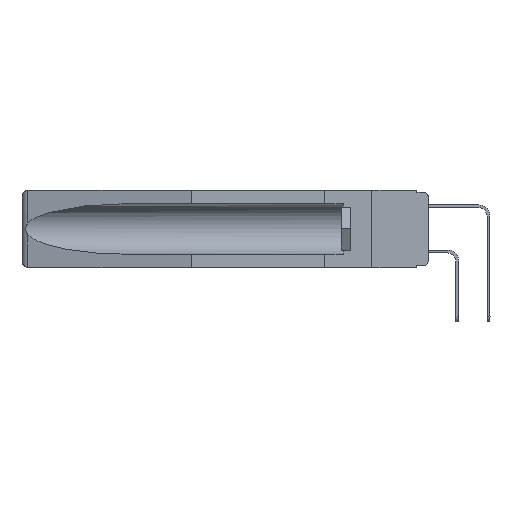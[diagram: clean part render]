
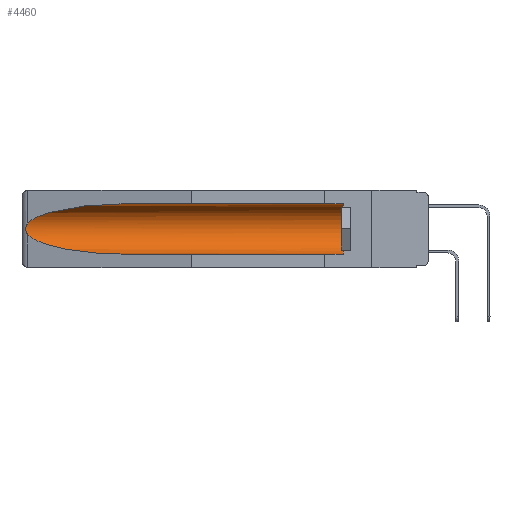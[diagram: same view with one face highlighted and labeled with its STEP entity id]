
A CAD part, left-side view. The second image highlights one B-rep face of the part: STEP entity #4460.
In plain terms, the highlighted cylindrical face has radius 2.857 mm (diameter 5.715 mm), a partial arc.
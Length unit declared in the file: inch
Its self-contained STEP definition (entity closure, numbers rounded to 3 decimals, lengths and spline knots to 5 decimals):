
#137 = DIRECTION ( 'NONE',  ( 0., -1., 0. ) ) ;
#471 = CARTESIAN_POINT ( 'NONE',  ( 0.2675, 1.53308, -0.17534 ) ) ;
#1247 = CARTESIAN_POINT ( 'NONE',  ( 0.25451, 1.48313, -0.24835 ) ) ;
#1530 = LINE ( 'NONE', #14724, #13781 ) ;
#1669 = CARTESIAN_POINT ( 'NONE',  ( 0.155, 0.126, -0.284 ) ) ;
#1723 = CARTESIAN_POINT ( 'NONE',  ( 0.2673, 1.53269, -0.17917 ) ) ;
#2307 = ORIENTED_EDGE ( 'NONE', *, *, #15177, .T. ) ;
#2541 = VERTEX_POINT ( 'NONE', #2817 ) ;
#2593 = VERTEX_POINT ( 'NONE', #18043 ) ;
#2817 = CARTESIAN_POINT ( 'NONE',  ( 0.26537, 1.52718, -0.14972 ) ) ;
#3163 = ORIENTED_EDGE ( 'NONE', *, *, #12112, .T. ) ;
#3260 = CARTESIAN_POINT ( 'NONE',  ( 0.155, 1.07973, -0.284 ) ) ;
#3589 = CYLINDRICAL_SURFACE ( 'NONE', #11812, 0.1125 ) ;
#3646 = CARTESIAN_POINT ( 'NONE',  ( 0.26597, 1.52961, -0.15275 ) ) ;
#3725 = ORIENTED_EDGE ( 'NONE', *, *, #11303, .T. ) ;
#4099 = CARTESIAN_POINT ( 'NONE',  ( 0.155, 1.07973, -0.059 ) ) ;
#4169 = EDGE_CURVE ( 'NONE', #15071, #11388, #14285, .T. ) ;
#4353 = AXIS2_PLACEMENT_3D ( 'NONE', #7747, #137, #16620 ) ;
#4460 = ADVANCED_FACE ( 'NONE', ( #13708 ), #3589, .F. ) ;
#4886 = CARTESIAN_POINT ( 'NONE',  ( 0.26537, 1.52718, -0.14972 ) ) ;
#4989 = CARTESIAN_POINT ( 'NONE',  ( 0.2675, 1.53308, -0.16763 ) ) ;
#5112 = EDGE_CURVE ( 'NONE', #15531, #12094, #1530, .T. ) ;
#5751 = DIRECTION ( 'NONE',  ( 0., 1., 0. ) ) ;
#5797 = CARTESIAN_POINT ( 'NONE',  ( 0.155, -0.30754, -0.284 ) ) ;
#6389 = CARTESIAN_POINT ( 'NONE',  ( 0.155, 1.07973, -0.059 ) ) ;
#6441 = CARTESIAN_POINT ( 'NONE',  ( 0.26654, 1.53092, -0.15636 ) ) ;
#6485 =( BOUNDED_CURVE ( )  B_SPLINE_CURVE ( 3, ( #4099, #12782, #17315, #12501 ),
 .UNSPECIFIED., .F., .F. ) 
 B_SPLINE_CURVE_WITH_KNOTS ( ( 4, 4 ),
 ( 4.71239, 6.08839 ),
 .UNSPECIFIED. ) 
 CURVE ( )  GEOMETRIC_REPRESENTATION_ITEM ( )  RATIONAL_B_SPLINE_CURVE ( ( 1., 0.848, 0.848, 1. ) ) 
 REPRESENTATION_ITEM ( '' )  );
#6518 = CIRCLE ( 'NONE', #4353, 0.1125 ) ;
#6541 = CARTESIAN_POINT ( 'NONE',  ( 0.2673, 1.5327, -0.16383 ) ) ;
#6859 = EDGE_LOOP ( 'NONE', ( #13386, #3725, #2307, #12552, #3163, #13947 ) ) ;
#7354 = DIRECTION ( 'NONE',  ( 0., 1., 0. ) ) ;
#7615 = VECTOR ( 'NONE', #7354, 39.37008 ) ;
#7747 = CARTESIAN_POINT ( 'NONE',  ( 0.155, 0.126, -0.1715 ) ) ;
#7890 = CARTESIAN_POINT ( 'NONE',  ( 0.26597, 1.5296, -0.19026 ) ) ;
#8590 = CARTESIAN_POINT ( 'NONE',  ( 0.155, 0.126, -0.059 ) ) ;
#11303 = EDGE_CURVE ( 'NONE', #2541, #2593, #15389, .T. ) ;
#11388 = VERTEX_POINT ( 'NONE', #3260 ) ;
#11812 = AXIS2_PLACEMENT_3D ( 'NONE', #15251, #15345, #16895 ) ;
#12094 = VERTEX_POINT ( 'NONE', #6389 ) ;
#12112 = EDGE_CURVE ( 'NONE', #15071, #15531, #6518, .T. ) ;
#12426 = CARTESIAN_POINT ( 'NONE',  ( 0.26655, 1.53094, -0.18657 ) ) ;
#12501 = CARTESIAN_POINT ( 'NONE',  ( 0.26537, 1.52718, -0.14972 ) ) ;
#12552 = ORIENTED_EDGE ( 'NONE', *, *, #4169, .F. ) ;
#12782 = CARTESIAN_POINT ( 'NONE',  ( 0.21114, 1.30732, -0.059 ) ) ;
#13108 = CARTESIAN_POINT ( 'NONE',  ( 0.21114, 1.30732, -0.284 ) ) ;
#13386 = ORIENTED_EDGE ( 'NONE', *, *, #17619, .T. ) ;
#13708 = FACE_OUTER_BOUND ( 'NONE', #6859, .T. ) ;
#13781 = VECTOR ( 'NONE', #5751, 39.37008 ) ;
#13947 = ORIENTED_EDGE ( 'NONE', *, *, #5112, .T. ) ;
#14285 = LINE ( 'NONE', #5797, #7615 ) ;
#14724 = CARTESIAN_POINT ( 'NONE',  ( 0.155, -0.30754, -0.059 ) ) ;
#14831 = CARTESIAN_POINT ( 'NONE',  ( 0.155, 1.07973, -0.284 ) ) ;
#15071 = VERTEX_POINT ( 'NONE', #1669 ) ;
#15177 = EDGE_CURVE ( 'NONE', #2593, #11388, #17577, .T. ) ;
#15251 = CARTESIAN_POINT ( 'NONE',  ( 0.155, -0.30754, -0.1715 ) ) ;
#15345 = DIRECTION ( 'NONE',  ( 0., 1., 0. ) ) ;
#15389 = B_SPLINE_CURVE_WITH_KNOTS ( 'NONE', 3,
 ( #4886, #3646, #6441, #6541, #4989, #471, #1723, #12426, #7890, #18305 ),
 .UNSPECIFIED., .F., .F.,
 ( 4, 2, 2, 2, 4 ),
 ( 0., 0.00029, 0.00058, 0.00087, 0.00117 ),
 .UNSPECIFIED. ) ;
#15531 = VERTEX_POINT ( 'NONE', #8590 ) ;
#16620 = DIRECTION ( 'NONE',  ( 0., 0., 1. ) ) ;
#16895 = DIRECTION ( 'NONE',  ( 0., 0., 1. ) ) ;
#17315 = CARTESIAN_POINT ( 'NONE',  ( 0.25451, 1.48313, -0.09465 ) ) ;
#17577 =( BOUNDED_CURVE ( )  B_SPLINE_CURVE ( 3, ( #17726, #1247, #13108, #14831 ),
 .UNSPECIFIED., .F., .F. ) 
 B_SPLINE_CURVE_WITH_KNOTS ( ( 4, 4 ),
 ( 0.1948, 1.5708 ),
 .UNSPECIFIED. ) 
 CURVE ( )  GEOMETRIC_REPRESENTATION_ITEM ( )  RATIONAL_B_SPLINE_CURVE ( ( 1., 0.848, 0.848, 1. ) ) 
 REPRESENTATION_ITEM ( '' )  );
#17619 = EDGE_CURVE ( 'NONE', #12094, #2541, #6485, .T. ) ;
#17726 = CARTESIAN_POINT ( 'NONE',  ( 0.26537, 1.52718, -0.19328 ) ) ;
#18043 = CARTESIAN_POINT ( 'NONE',  ( 0.26537, 1.52718, -0.19328 ) ) ;
#18305 = CARTESIAN_POINT ( 'NONE',  ( 0.26537, 1.52718, -0.19328 ) ) ;
